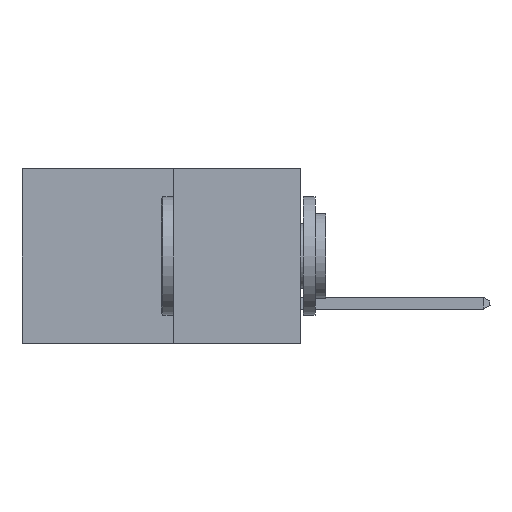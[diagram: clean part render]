
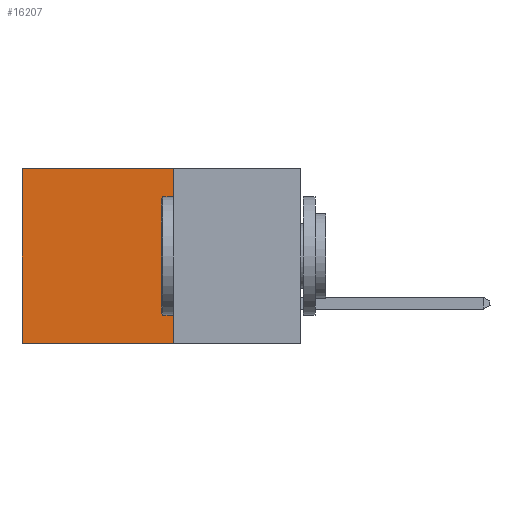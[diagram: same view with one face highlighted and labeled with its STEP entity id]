
A CAD part, left-side view. The second image highlights one B-rep face of the part: STEP entity #16207.
In plain terms, the highlighted planar face has unit normal (-1, 0, 0).
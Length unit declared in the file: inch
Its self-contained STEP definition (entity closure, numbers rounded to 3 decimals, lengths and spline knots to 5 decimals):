
#1194 = EDGE_CURVE ( 'NONE', #3852, #16386, #14980, .T. ) ;
#2021 = EDGE_CURVE ( 'NONE', #3852, #15986, #10521, .T. ) ;
#3049 = CARTESIAN_POINT ( 'NONE',  ( 0.277, 0.27, -0.37 ) ) ;
#3593 = CARTESIAN_POINT ( 'NONE',  ( 0.277, 0.27, -0.37 ) ) ;
#3852 = VERTEX_POINT ( 'NONE', #3920 ) ;
#3920 = CARTESIAN_POINT ( 'NONE',  ( 0.277, 0.27, 0. ) ) ;
#5133 = ORIENTED_EDGE ( 'NONE', *, *, #12071, .F. ) ;
#5172 = DIRECTION ( 'NONE',  ( 0., 0., -1. ) ) ;
#5596 = EDGE_LOOP ( 'NONE', ( #7879, #5133, #8018, #10282 ) ) ;
#5642 = AXIS2_PLACEMENT_3D ( 'NONE', #3593, #14171, #5172 ) ;
#6152 = CARTESIAN_POINT ( 'NONE',  ( 0.277, 0.59, 0. ) ) ;
#6504 = VECTOR ( 'NONE', #19186, 39.37008 ) ;
#6536 = CARTESIAN_POINT ( 'NONE',  ( 0.277, 0.59, -0.37 ) ) ;
#6551 = VECTOR ( 'NONE', #17312, 39.37008 ) ;
#7879 = ORIENTED_EDGE ( 'NONE', *, *, #9128, .T. ) ;
#8018 = ORIENTED_EDGE ( 'NONE', *, *, #1194, .F. ) ;
#9128 = EDGE_CURVE ( 'NONE', #15986, #14410, #19136, .T. ) ;
#9663 = PLANE ( 'NONE',  #5642 ) ;
#10282 = ORIENTED_EDGE ( 'NONE', *, *, #2021, .T. ) ;
#10521 = LINE ( 'NONE', #16066, #6504 ) ;
#10805 = LINE ( 'NONE', #3049, #14765 ) ;
#11244 = VECTOR ( 'NONE', #15511, 39.37008 ) ;
#12071 = EDGE_CURVE ( 'NONE', #16386, #14410, #10805, .T. ) ;
#14098 = FACE_OUTER_BOUND ( 'NONE', #5596, .T. ) ;
#14171 = DIRECTION ( 'NONE',  ( 1., 0., 0. ) ) ;
#14410 = VERTEX_POINT ( 'NONE', #17866 ) ;
#14765 = VECTOR ( 'NONE', #15129, 39.37008 ) ;
#14980 = LINE ( 'NONE', #19333, #6551 ) ;
#15129 = DIRECTION ( 'NONE',  ( 0., 1., 0. ) ) ;
#15511 = DIRECTION ( 'NONE',  ( 0., 0., -1. ) ) ;
#15986 = VERTEX_POINT ( 'NONE', #6152 ) ;
#15998 = CARTESIAN_POINT ( 'NONE',  ( 0.277, 0.27, -0.37 ) ) ;
#16066 = CARTESIAN_POINT ( 'NONE',  ( 0.277, 0.27, 0. ) ) ;
#16207 = ADVANCED_FACE ( 'NONE', ( #14098 ), #9663, .F. ) ;
#16386 = VERTEX_POINT ( 'NONE', #15998 ) ;
#17312 = DIRECTION ( 'NONE',  ( 0., 0., -1. ) ) ;
#17866 = CARTESIAN_POINT ( 'NONE',  ( 0.277, 0.59, -0.37 ) ) ;
#19136 = LINE ( 'NONE', #6536, #11244 ) ;
#19186 = DIRECTION ( 'NONE',  ( 0., 1., 0. ) ) ;
#19333 = CARTESIAN_POINT ( 'NONE',  ( 0.277, 0.27, -0.37 ) ) ;
